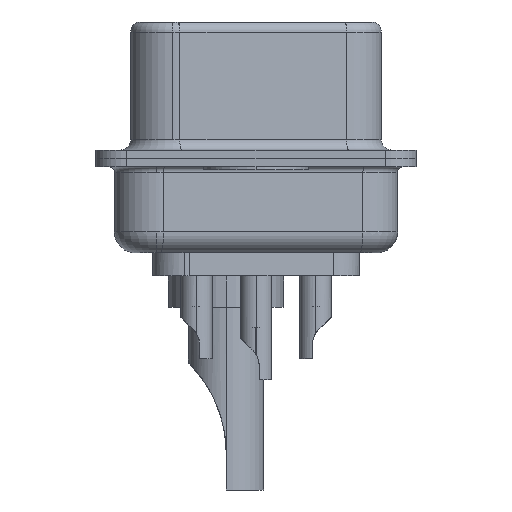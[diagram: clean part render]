
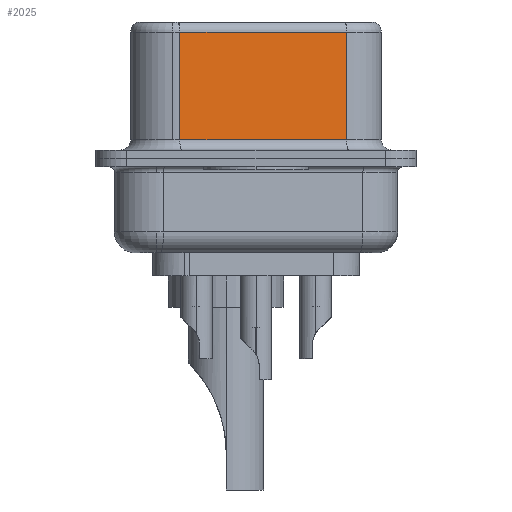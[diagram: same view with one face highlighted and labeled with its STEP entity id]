
A CAD part, left-side view. The second image highlights one B-rep face of the part: STEP entity #2025.
In plain terms, the highlighted planar face has unit normal (-0.985, -0.174, 0).
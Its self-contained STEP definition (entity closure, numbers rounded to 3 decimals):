
#115 = ORIENTED_EDGE ( 'NONE', *, *, #21129, .T. ) ;
#154 = VECTOR ( 'NONE', #22460, 1000. ) ;
#1713 = CARTESIAN_POINT ( 'NONE',  ( 5.132, -4.322, 0.9 ) ) ;
#2025 = ADVANCED_FACE ( 'NONE', ( #12872 ), #16491, .F. ) ;
#2171 = VECTOR ( 'NONE', #10207, 1000. ) ;
#2644 = CARTESIAN_POINT ( 'NONE',  ( 3.73, 3.628, 6.52 ) ) ;
#2798 = EDGE_CURVE ( 'NONE', #18222, #6281, #15117, .T. ) ;
#3104 = LINE ( 'NONE', #2644, #18398 ) ;
#4120 = VERTEX_POINT ( 'NONE', #19035 ) ;
#4726 = DIRECTION ( 'NONE',  ( 0., 0., -1. ) ) ;
#4846 = CARTESIAN_POINT ( 'NONE',  ( 5.132, -4.322, 0.9 ) ) ;
#6281 = VERTEX_POINT ( 'NONE', #1713 ) ;
#8315 = EDGE_LOOP ( 'NONE', ( #26667, #15331, #8398, #115 ) ) ;
#8398 = ORIENTED_EDGE ( 'NONE', *, *, #23665, .T. ) ;
#9951 = AXIS2_PLACEMENT_3D ( 'NONE', #26914, #26387, #17534 ) ;
#10207 = DIRECTION ( 'NONE',  ( 0., 0., -1. ) ) ;
#10563 = VECTOR ( 'NONE', #11040, 1000. ) ;
#11040 = DIRECTION ( 'NONE',  ( 0.174, -0.985, 0. ) ) ;
#11919 = CARTESIAN_POINT ( 'NONE',  ( 3.73, 3.628, 6.02 ) ) ;
#11944 = CARTESIAN_POINT ( 'NONE',  ( 5.132, -4.322, 6.02 ) ) ;
#12872 = FACE_OUTER_BOUND ( 'NONE', #8315, .T. ) ;
#15117 = LINE ( 'NONE', #25513, #2171 ) ;
#15331 = ORIENTED_EDGE ( 'NONE', *, *, #24013, .T. ) ;
#16491 = PLANE ( 'NONE',  #9951 ) ;
#16551 = VERTEX_POINT ( 'NONE', #11919 ) ;
#17534 = DIRECTION ( 'NONE',  ( -0.174, 0.985, 0. ) ) ;
#18222 = VERTEX_POINT ( 'NONE', #11944 ) ;
#18247 = CARTESIAN_POINT ( 'NONE',  ( 5.132, -4.322, 6.02 ) ) ;
#18398 = VECTOR ( 'NONE', #4726, 1000. ) ;
#19035 = CARTESIAN_POINT ( 'NONE',  ( 3.73, 3.628, 0.9 ) ) ;
#21129 = EDGE_CURVE ( 'NONE', #4120, #6281, #21689, .T. ) ;
#21689 = LINE ( 'NONE', #4846, #10563 ) ;
#22460 = DIRECTION ( 'NONE',  ( -0.174, 0.985, 0. ) ) ;
#22944 = LINE ( 'NONE', #18247, #154 ) ;
#23665 = EDGE_CURVE ( 'NONE', #16551, #4120, #3104, .T. ) ;
#24013 = EDGE_CURVE ( 'NONE', #18222, #16551, #22944, .T. ) ;
#25513 = CARTESIAN_POINT ( 'NONE',  ( 5.132, -4.322, 6.52 ) ) ;
#26387 = DIRECTION ( 'NONE',  ( 0.985, 0.174, 0. ) ) ;
#26667 = ORIENTED_EDGE ( 'NONE', *, *, #2798, .F. ) ;
#26914 = CARTESIAN_POINT ( 'NONE',  ( 5.132, -4.322, 6.52 ) ) ;
